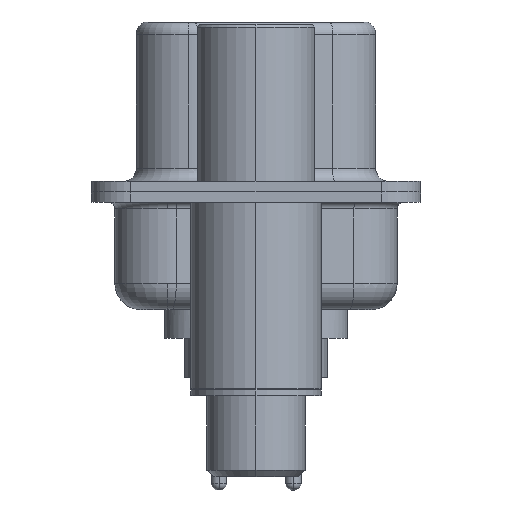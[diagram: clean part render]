
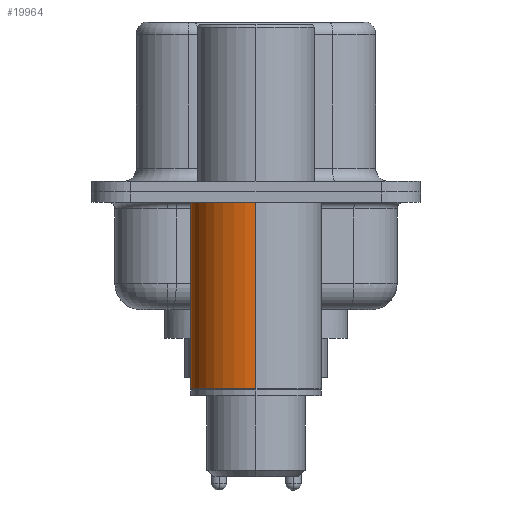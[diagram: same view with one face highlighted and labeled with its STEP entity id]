
A CAD part, left-side view. The second image highlights one B-rep face of the part: STEP entity #19964.
In plain terms, the highlighted cylindrical face has radius 2.5 mm (diameter 5 mm), a partial arc.
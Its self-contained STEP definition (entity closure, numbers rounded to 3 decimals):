
#230 = EDGE_CURVE ( 'NONE', #19160, #3385, #15038, .T. ) ;
#294 = AXIS2_PLACEMENT_3D ( 'NONE', #10578, #11075, #11804 ) ;
#308 = DIRECTION ( 'NONE',  ( 0., 0., 1. ) ) ;
#1179 = CARTESIAN_POINT ( 'NONE',  ( 2.5, 0., -0.4 ) ) ;
#1240 = EDGE_CURVE ( 'NONE', #19160, #5740, #9470, .T. ) ;
#3385 = VERTEX_POINT ( 'NONE', #17439 ) ;
#3648 = DIRECTION ( 'NONE',  ( 0., 0., 1. ) ) ;
#4158 = DIRECTION ( 'NONE',  ( 0., 0., 1. ) ) ;
#5740 = VERTEX_POINT ( 'NONE', #1179 ) ;
#5958 = CARTESIAN_POINT ( 'NONE',  ( 2.5, 0., 0.581 ) ) ;
#6908 = EDGE_CURVE ( 'NONE', #3385, #10782, #18103, .T. ) ;
#7009 = CYLINDRICAL_SURFACE ( 'NONE', #7513, 2.5 ) ;
#7513 = AXIS2_PLACEMENT_3D ( 'NONE', #17699, #3648, #8301 ) ;
#8128 = CARTESIAN_POINT ( 'NONE',  ( -2.5, 0., -0.4 ) ) ;
#8301 = DIRECTION ( 'NONE',  ( 1., 0., 0. ) ) ;
#8979 = VECTOR ( 'NONE', #14833, 1000. ) ;
#9470 = LINE ( 'NONE', #5958, #8979 ) ;
#9646 = CARTESIAN_POINT ( 'NONE',  ( 0., 0., -0.4 ) ) ;
#10578 = CARTESIAN_POINT ( 'NONE',  ( 0., 0., -7.525 ) ) ;
#10782 = VERTEX_POINT ( 'NONE', #8128 ) ;
#11075 = DIRECTION ( 'NONE',  ( 0., 0., 1. ) ) ;
#11243 = DIRECTION ( 'NONE',  ( 1., 0., 0. ) ) ;
#11448 = EDGE_CURVE ( 'NONE', #5740, #10782, #18053, .T. ) ;
#11804 = DIRECTION ( 'NONE',  ( 1., 0., 0. ) ) ;
#12398 = CARTESIAN_POINT ( 'NONE',  ( 2.5, 0., -7.525 ) ) ;
#13147 = AXIS2_PLACEMENT_3D ( 'NONE', #9646, #308, #11243 ) ;
#13625 = CARTESIAN_POINT ( 'NONE',  ( -2.5, 0., 0.581 ) ) ;
#14833 = DIRECTION ( 'NONE',  ( 0., 0., 1. ) ) ;
#14945 = EDGE_LOOP ( 'NONE', ( #16816, #16069, #15248, #17890 ) ) ;
#15038 = CIRCLE ( 'NONE', #294, 2.5 ) ;
#15248 = ORIENTED_EDGE ( 'NONE', *, *, #11448, .F. ) ;
#15344 = FACE_OUTER_BOUND ( 'NONE', #14945, .T. ) ;
#16069 = ORIENTED_EDGE ( 'NONE', *, *, #6908, .T. ) ;
#16816 = ORIENTED_EDGE ( 'NONE', *, *, #230, .T. ) ;
#17439 = CARTESIAN_POINT ( 'NONE',  ( -2.5, 0., -7.525 ) ) ;
#17699 = CARTESIAN_POINT ( 'NONE',  ( 0., 0., 0.581 ) ) ;
#17890 = ORIENTED_EDGE ( 'NONE', *, *, #1240, .F. ) ;
#18053 = CIRCLE ( 'NONE', #13147, 2.5 ) ;
#18103 = LINE ( 'NONE', #13625, #18579 ) ;
#18579 = VECTOR ( 'NONE', #4158, 1000. ) ;
#19160 = VERTEX_POINT ( 'NONE', #12398 ) ;
#19964 = ADVANCED_FACE ( 'NONE', ( #15344 ), #7009, .T. ) ;
